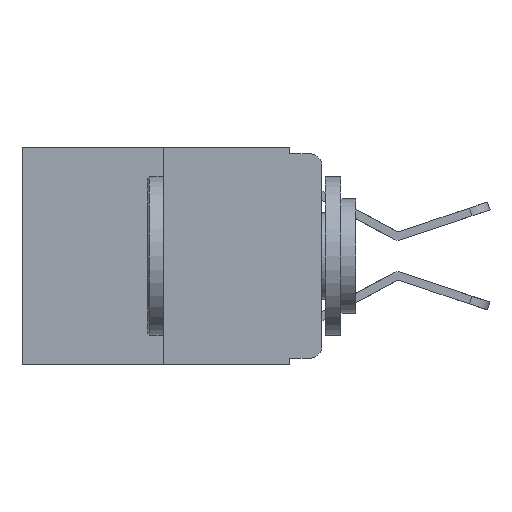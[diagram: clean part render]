
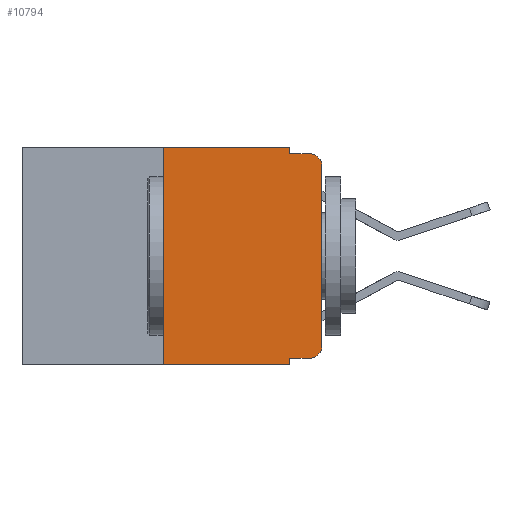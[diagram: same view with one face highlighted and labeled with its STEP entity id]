
A CAD part, left-side view. The second image highlights one B-rep face of the part: STEP entity #10794.
In plain terms, the highlighted planar face has unit normal (-1, 0, 0).
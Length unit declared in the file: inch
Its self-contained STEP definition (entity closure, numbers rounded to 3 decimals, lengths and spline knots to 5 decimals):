
#46 = ORIENTED_EDGE ( 'NONE', *, *, #11765, .T. ) ;
#96 = DIRECTION ( 'NONE',  ( 0., 0., -1. ) ) ;
#218 = VERTEX_POINT ( 'NONE', #6809 ) ;
#350 = VECTOR ( 'NONE', #96, 39.37008 ) ;
#419 = EDGE_CURVE ( 'NONE', #4201, #8428, #8126, .T. ) ;
#873 = ORIENTED_EDGE ( 'NONE', *, *, #2724, .T. ) ;
#918 = VECTOR ( 'NONE', #7758, 39.37008 ) ;
#1004 = AXIS2_PLACEMENT_3D ( 'NONE', #12752, #13058, #13904 ) ;
#1126 = VERTEX_POINT ( 'NONE', #12491 ) ;
#1130 = CARTESIAN_POINT ( 'NONE',  ( 0., 0.02, -0.313 ) ) ;
#1230 = VERTEX_POINT ( 'NONE', #1971 ) ;
#1236 = EDGE_CURVE ( 'NONE', #5904, #8428, #9776, .T. ) ;
#1339 = DIRECTION ( 'NONE',  ( 0., 0., 1. ) ) ;
#1358 = FACE_OUTER_BOUND ( 'NONE', #2831, .T. ) ;
#1661 = CARTESIAN_POINT ( 'NONE',  ( 0., 0.051, -0.333 ) ) ;
#1971 = CARTESIAN_POINT ( 'NONE',  ( 0., 0.25, -0.343 ) ) ;
#2241 = DIRECTION ( 'NONE',  ( 0., 0., -1. ) ) ;
#2340 = DIRECTION ( 'NONE',  ( 0., -1., 0. ) ) ;
#2405 = VERTEX_POINT ( 'NONE', #12640 ) ;
#2724 = EDGE_CURVE ( 'NONE', #7613, #5904, #4885, .T. ) ;
#2727 = DIRECTION ( 'NONE',  ( 0., -1., 0. ) ) ;
#2782 = DIRECTION ( 'NONE',  ( 1., 0., 0. ) ) ;
#2793 = LINE ( 'NONE', #6927, #11222 ) ;
#2831 = EDGE_LOOP ( 'NONE', ( #873, #10438, #8300, #6725, #10620, #2934, #11981, #12588, #46, #12753 ) ) ;
#2934 = ORIENTED_EDGE ( 'NONE', *, *, #13083, .F. ) ;
#3013 = LINE ( 'NONE', #3584, #350 ) ;
#3224 = LINE ( 'NONE', #9114, #9209 ) ;
#3424 = CIRCLE ( 'NONE', #11411, 0.02 ) ;
#3584 = CARTESIAN_POINT ( 'NONE',  ( 0., 0.051, 0. ) ) ;
#3848 = CARTESIAN_POINT ( 'NONE',  ( 0., 0.473, 0. ) ) ;
#3891 = LINE ( 'NONE', #10947, #918 ) ;
#4201 = VERTEX_POINT ( 'NONE', #5810 ) ;
#4885 = LINE ( 'NONE', #6006, #5246 ) ;
#5132 = VECTOR ( 'NONE', #9059, 39.37008 ) ;
#5246 = VECTOR ( 'NONE', #5710, 39.37008 ) ;
#5505 = VECTOR ( 'NONE', #1339, 39.37008 ) ;
#5710 = DIRECTION ( 'NONE',  ( 0., 0., 1. ) ) ;
#5810 = CARTESIAN_POINT ( 'NONE',  ( 0., 0.051, -0.01 ) ) ;
#5828 = CARTESIAN_POINT ( 'NONE',  ( 0., 0.25, 0. ) ) ;
#5904 = VERTEX_POINT ( 'NONE', #8299 ) ;
#6006 = CARTESIAN_POINT ( 'NONE',  ( 0., 0., 0. ) ) ;
#6161 = PLANE ( 'NONE',  #7446 ) ;
#6617 = EDGE_CURVE ( 'NONE', #2405, #218, #8447, .T. ) ;
#6725 = ORIENTED_EDGE ( 'NONE', *, *, #13724, .F. ) ;
#6809 = CARTESIAN_POINT ( 'NONE',  ( 0., 0.051, 0. ) ) ;
#6927 = CARTESIAN_POINT ( 'NONE',  ( 0., 0.473, -0.343 ) ) ;
#7446 = AXIS2_PLACEMENT_3D ( 'NONE', #9495, #2782, #10532 ) ;
#7613 = VERTEX_POINT ( 'NONE', #10740 ) ;
#7758 = DIRECTION ( 'NONE',  ( 0., 0., -1. ) ) ;
#7906 = CARTESIAN_POINT ( 'NONE',  ( 0., 0.02, -0.333 ) ) ;
#8039 = DIRECTION ( 'NONE',  ( 0., -1., 0. ) ) ;
#8126 = LINE ( 'NONE', #12022, #5132 ) ;
#8299 = CARTESIAN_POINT ( 'NONE',  ( 0., 0., -0.03 ) ) ;
#8300 = ORIENTED_EDGE ( 'NONE', *, *, #419, .F. ) ;
#8428 = VERTEX_POINT ( 'NONE', #9014 ) ;
#8447 = LINE ( 'NONE', #3848, #8790 ) ;
#8494 = LINE ( 'NONE', #5828, #5505 ) ;
#8496 = EDGE_CURVE ( 'NONE', #1230, #1126, #2793, .T. ) ;
#8790 = VECTOR ( 'NONE', #2727, 39.37008 ) ;
#8988 = DIRECTION ( 'NONE',  ( -1., 0., 0. ) ) ;
#9014 = CARTESIAN_POINT ( 'NONE',  ( 0., 0.02, -0.01 ) ) ;
#9059 = DIRECTION ( 'NONE',  ( 0., -1., 0. ) ) ;
#9114 = CARTESIAN_POINT ( 'NONE',  ( 0., 0.051, -0.333 ) ) ;
#9209 = VECTOR ( 'NONE', #2340, 39.37008 ) ;
#9495 = CARTESIAN_POINT ( 'NONE',  ( 0., 0.473, 0. ) ) ;
#9601 = VERTEX_POINT ( 'NONE', #7906 ) ;
#9776 = CIRCLE ( 'NONE', #1004, 0.02 ) ;
#9928 = VERTEX_POINT ( 'NONE', #1661 ) ;
#10438 = ORIENTED_EDGE ( 'NONE', *, *, #1236, .T. ) ;
#10532 = DIRECTION ( 'NONE',  ( 0., 0., -1. ) ) ;
#10620 = ORIENTED_EDGE ( 'NONE', *, *, #6617, .F. ) ;
#10740 = CARTESIAN_POINT ( 'NONE',  ( 0., 0., -0.313 ) ) ;
#10794 = ADVANCED_FACE ( 'NONE', ( #1358 ), #6161, .F. ) ;
#10947 = CARTESIAN_POINT ( 'NONE',  ( 0., 0.051, 0. ) ) ;
#11102 = EDGE_CURVE ( 'NONE', #9601, #7613, #3424, .T. ) ;
#11222 = VECTOR ( 'NONE', #8039, 39.37008 ) ;
#11411 = AXIS2_PLACEMENT_3D ( 'NONE', #1130, #8988, #2241 ) ;
#11765 = EDGE_CURVE ( 'NONE', #9928, #9601, #3224, .T. ) ;
#11981 = ORIENTED_EDGE ( 'NONE', *, *, #8496, .T. ) ;
#12022 = CARTESIAN_POINT ( 'NONE',  ( 0., 0.051, -0.01 ) ) ;
#12419 = EDGE_CURVE ( 'NONE', #9928, #1126, #3013, .T. ) ;
#12491 = CARTESIAN_POINT ( 'NONE',  ( 0., 0.051, -0.343 ) ) ;
#12588 = ORIENTED_EDGE ( 'NONE', *, *, #12419, .F. ) ;
#12640 = CARTESIAN_POINT ( 'NONE',  ( 0., 0.25, 0. ) ) ;
#12752 = CARTESIAN_POINT ( 'NONE',  ( 0., 0.02, -0.03 ) ) ;
#12753 = ORIENTED_EDGE ( 'NONE', *, *, #11102, .T. ) ;
#13058 = DIRECTION ( 'NONE',  ( -1., 0., 0. ) ) ;
#13083 = EDGE_CURVE ( 'NONE', #1230, #2405, #8494, .T. ) ;
#13724 = EDGE_CURVE ( 'NONE', #218, #4201, #3891, .T. ) ;
#13904 = DIRECTION ( 'NONE',  ( 0., 0., -1. ) ) ;
